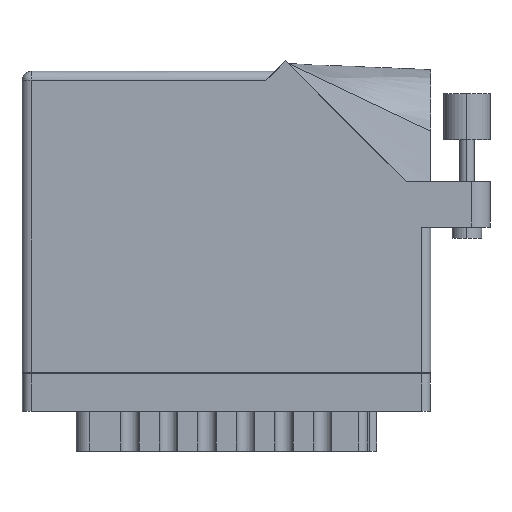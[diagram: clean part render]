
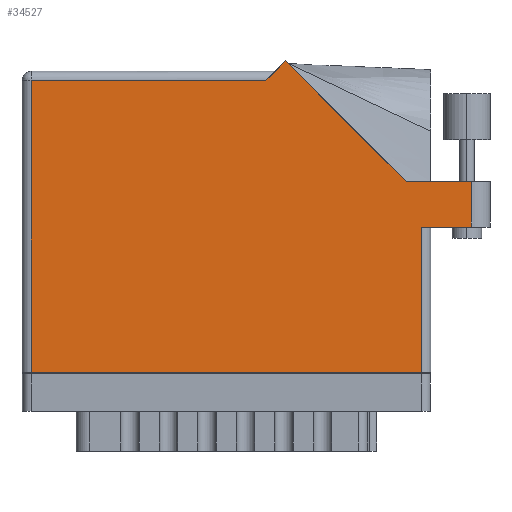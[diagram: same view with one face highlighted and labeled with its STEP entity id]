
A CAD part, front view. The second image highlights one B-rep face of the part: STEP entity #34527.
In plain terms, the highlighted face is planar.
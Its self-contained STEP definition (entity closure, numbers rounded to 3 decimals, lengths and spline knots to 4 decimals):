
#977 = CARTESIAN_POINT ( 'NONE',  ( 3.03, 0.98, 0. ) ) ;
#4203 = DIRECTION ( 'NONE',  ( -0.707, 0.707, 0. ) ) ;
#4272 = DIRECTION ( 'NONE',  ( 0., 1., 0. ) ) ;
#6128 = LINE ( 'NONE', #34391, #47870 ) ;
#6579 = AXIS2_PLACEMENT_3D ( 'NONE', #77571, #45149, #64063 ) ;
#7225 = DIRECTION ( 'NONE',  ( -1., 0., 0. ) ) ;
#7826 = LINE ( 'NONE', #72253, #12033 ) ;
#9706 = CARTESIAN_POINT ( 'NONE',  ( 2.5894, 1.287, 0. ) ) ;
#10022 = CARTESIAN_POINT ( 'NONE',  ( 2.5894, 1.287, 0. ) ) ;
#10508 = CARTESIAN_POINT ( 'NONE',  ( 0.062, 0., 0. ) ) ;
#10689 = EDGE_CURVE ( 'NONE', #81581, #12598, #6128, .T. ) ;
#11499 = ORIENTED_EDGE ( 'NONE', *, *, #65133, .T. ) ;
#12033 = VECTOR ( 'NONE', #52653, 39.3701 ) ;
#12598 = VERTEX_POINT ( 'NONE', #51583 ) ;
#15474 = LINE ( 'NONE', #34617, #84360 ) ;
#17001 = DIRECTION ( 'NONE',  ( 1., 0., 0. ) ) ;
#24176 = PLANE ( 'NONE',  #6579 ) ;
#24307 = VERTEX_POINT ( 'NONE', #9706 ) ;
#24394 = EDGE_CURVE ( 'NONE', #41437, #48533, #44472, .T. ) ;
#24403 = ORIENTED_EDGE ( 'NONE', *, *, #55324, .T. ) ;
#24760 = VERTEX_POINT ( 'NONE', #41761 ) ;
#26408 = CARTESIAN_POINT ( 'NONE',  ( 0.062, 1.968, 0. ) ) ;
#26837 = LINE ( 'NONE', #77476, #86333 ) ;
#28932 = EDGE_LOOP ( 'NONE', ( #66768, #32346, #74661, #83094, #33395, #34265, #24403, #11499, #71492 ) ) ;
#30038 = VERTEX_POINT ( 'NONE', #10508 ) ;
#30437 = VECTOR ( 'NONE', #55916, 39.3701 ) ;
#31486 = LINE ( 'NONE', #61776, #30437 ) ;
#32035 = EDGE_CURVE ( 'NONE', #48533, #24760, #77470, .T. ) ;
#32346 = ORIENTED_EDGE ( 'NONE', *, *, #32035, .T. ) ;
#33395 = ORIENTED_EDGE ( 'NONE', *, *, #10689, .T. ) ;
#34265 = ORIENTED_EDGE ( 'NONE', *, *, #37789, .T. ) ;
#34391 = CARTESIAN_POINT ( 'NONE',  ( 1.705, 2.03, 0. ) ) ;
#34527 = ADVANCED_FACE ( 'NONE', ( #38489 ), #24176, .F. ) ;
#34617 = CARTESIAN_POINT ( 'NONE',  ( 3.155, 1.287, 0. ) ) ;
#37413 = CARTESIAN_POINT ( 'NONE',  ( 2.755, 0.98, 0. ) ) ;
#37789 = EDGE_CURVE ( 'NONE', #12598, #84918, #43294, .T. ) ;
#38489 = FACE_OUTER_BOUND ( 'NONE', #28932, .T. ) ;
#38711 = CARTESIAN_POINT ( 'NONE',  ( 2.693, 0., 0. ) ) ;
#40825 = VECTOR ( 'NONE', #4203, 39.3701 ) ;
#41437 = VERTEX_POINT ( 'NONE', #65969 ) ;
#41761 = CARTESIAN_POINT ( 'NONE',  ( 3.03, 1.287, 0. ) ) ;
#43294 = LINE ( 'NONE', #63988, #83010 ) ;
#43469 = VECTOR ( 'NONE', #17001, 39.3701 ) ;
#44472 = LINE ( 'NONE', #37413, #43469 ) ;
#45149 = DIRECTION ( 'NONE',  ( 0., 0., -1. ) ) ;
#47870 = VECTOR ( 'NONE', #82852, 39.3701 ) ;
#47915 = CARTESIAN_POINT ( 'NONE',  ( 3.03, 1.287, 0. ) ) ;
#48533 = VERTEX_POINT ( 'NONE', #977 ) ;
#51583 = CARTESIAN_POINT ( 'NONE',  ( 1.643, 1.968, 0. ) ) ;
#52653 = DIRECTION ( 'NONE',  ( 0., -1., 0. ) ) ;
#55324 = EDGE_CURVE ( 'NONE', #84918, #30038, #7826, .T. ) ;
#55916 = DIRECTION ( 'NONE',  ( 1., 0., 0. ) ) ;
#61776 = CARTESIAN_POINT ( 'NONE',  ( 0., 0., 0. ) ) ;
#62177 = DIRECTION ( 'NONE',  ( 0., 1., 0. ) ) ;
#63988 = CARTESIAN_POINT ( 'NONE',  ( 0., 1.968, 0. ) ) ;
#64063 = DIRECTION ( 'NONE',  ( -1., 0., 0. ) ) ;
#65133 = EDGE_CURVE ( 'NONE', #30038, #66908, #31486, .T. ) ;
#65683 = EDGE_CURVE ( 'NONE', #24307, #81581, #78401, .T. ) ;
#65969 = CARTESIAN_POINT ( 'NONE',  ( 2.693, 0.98, 0. ) ) ;
#66768 = ORIENTED_EDGE ( 'NONE', *, *, #24394, .T. ) ;
#66908 = VERTEX_POINT ( 'NONE', #38711 ) ;
#70577 = CARTESIAN_POINT ( 'NONE',  ( 1.7757, 2.1007, 0. ) ) ;
#71492 = ORIENTED_EDGE ( 'NONE', *, *, #83098, .T. ) ;
#72253 = CARTESIAN_POINT ( 'NONE',  ( 0.062, 0., 0. ) ) ;
#74661 = ORIENTED_EDGE ( 'NONE', *, *, #82806, .T. ) ;
#77470 = LINE ( 'NONE', #47915, #78472 ) ;
#77476 = CARTESIAN_POINT ( 'NONE',  ( 2.693, 0.98, 0. ) ) ;
#77571 = CARTESIAN_POINT ( 'NONE',  ( 0., 2.03, 0. ) ) ;
#78401 = LINE ( 'NONE', #10022, #40825 ) ;
#78472 = VECTOR ( 'NONE', #62177, 39.3701 ) ;
#81581 = VERTEX_POINT ( 'NONE', #70577 ) ;
#82806 = EDGE_CURVE ( 'NONE', #24760, #24307, #15474, .T. ) ;
#82852 = DIRECTION ( 'NONE',  ( -0.707, -0.707, 0. ) ) ;
#83010 = VECTOR ( 'NONE', #83948, 39.3701 ) ;
#83094 = ORIENTED_EDGE ( 'NONE', *, *, #65683, .T. ) ;
#83098 = EDGE_CURVE ( 'NONE', #66908, #41437, #26837, .T. ) ;
#83948 = DIRECTION ( 'NONE',  ( -1., 0., 0. ) ) ;
#84360 = VECTOR ( 'NONE', #7225, 39.3701 ) ;
#84918 = VERTEX_POINT ( 'NONE', #26408 ) ;
#86333 = VECTOR ( 'NONE', #4272, 39.3701 ) ;
